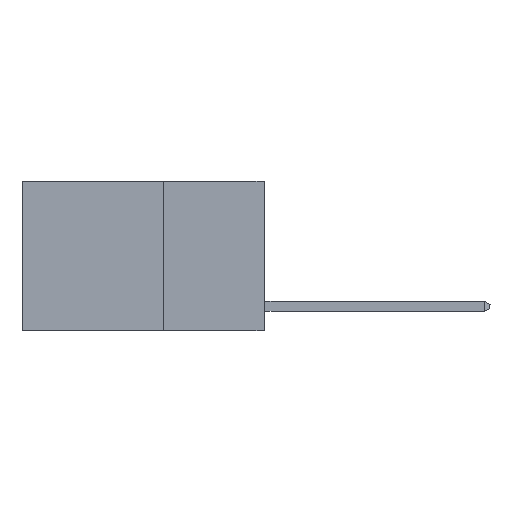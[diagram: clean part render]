
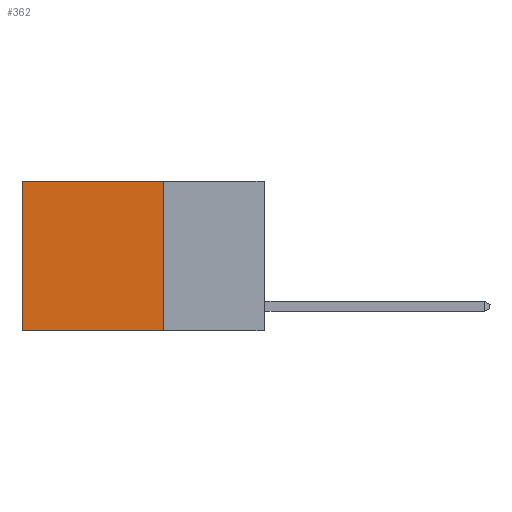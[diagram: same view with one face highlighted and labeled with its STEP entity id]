
A CAD part, left-side view. The second image highlights one B-rep face of the part: STEP entity #362.
In plain terms, the highlighted planar face has unit normal (-1, 0, 0).
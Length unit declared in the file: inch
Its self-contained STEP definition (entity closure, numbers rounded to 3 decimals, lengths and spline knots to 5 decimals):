
#362 = ADVANCED_FACE ( 'NONE', ( #10536 ), #10525, .F. ) ;
#374 = VECTOR ( 'NONE', #8111, 39.37008 ) ;
#999 = VECTOR ( 'NONE', #11682, 39.37008 ) ;
#1847 = ORIENTED_EDGE ( 'NONE', *, *, #6568, .F. ) ;
#2154 = CARTESIAN_POINT ( 'NONE',  ( 0.2625, 0.25, 0. ) ) ;
#2304 = EDGE_CURVE ( 'NONE', #8043, #5341, #3570, .T. ) ;
#2521 = AXIS2_PLACEMENT_3D ( 'NONE', #8917, #4760, #12077 ) ;
#2674 = EDGE_LOOP ( 'NONE', ( #4065, #3410, #1847, #13444 ) ) ;
#3410 = ORIENTED_EDGE ( 'NONE', *, *, #8800, .F. ) ;
#3570 = LINE ( 'NONE', #11479, #9273 ) ;
#4065 = ORIENTED_EDGE ( 'NONE', *, *, #2304, .T. ) ;
#4760 = DIRECTION ( 'NONE',  ( 1., 0., 0. ) ) ;
#5081 = VERTEX_POINT ( 'NONE', #11031 ) ;
#5341 = VERTEX_POINT ( 'NONE', #13574 ) ;
#6568 = EDGE_CURVE ( 'NONE', #11710, #5081, #12863, .T. ) ;
#6842 = CARTESIAN_POINT ( 'NONE',  ( 0.2625, 0.6, 0. ) ) ;
#6962 = CARTESIAN_POINT ( 'NONE',  ( 0.2625, 0.25, 0. ) ) ;
#8043 = VERTEX_POINT ( 'NONE', #6842 ) ;
#8111 = DIRECTION ( 'NONE',  ( 0., 1., 0. ) ) ;
#8800 = EDGE_CURVE ( 'NONE', #5081, #5341, #10043, .T. ) ;
#8917 = CARTESIAN_POINT ( 'NONE',  ( 0.2625, 0.25, 0. ) ) ;
#9273 = VECTOR ( 'NONE', #11380, 39.37008 ) ;
#9442 = LINE ( 'NONE', #6962, #374 ) ;
#10043 = LINE ( 'NONE', #10584, #999 ) ;
#10317 = VECTOR ( 'NONE', #13402, 39.37008 ) ;
#10525 = PLANE ( 'NONE',  #2521 ) ;
#10536 = FACE_OUTER_BOUND ( 'NONE', #2674, .T. ) ;
#10584 = CARTESIAN_POINT ( 'NONE',  ( 0.2625, 0.25, -0.37 ) ) ;
#11031 = CARTESIAN_POINT ( 'NONE',  ( 0.2625, 0.25, -0.37 ) ) ;
#11201 = EDGE_CURVE ( 'NONE', #11710, #8043, #9442, .T. ) ;
#11380 = DIRECTION ( 'NONE',  ( 0., 0., -1. ) ) ;
#11479 = CARTESIAN_POINT ( 'NONE',  ( 0.2625, 0.6, 0. ) ) ;
#11682 = DIRECTION ( 'NONE',  ( 0., 1., 0. ) ) ;
#11710 = VERTEX_POINT ( 'NONE', #2154 ) ;
#12077 = DIRECTION ( 'NONE',  ( 0., 0., -1. ) ) ;
#12367 = CARTESIAN_POINT ( 'NONE',  ( 0.2625, 0.25, 0. ) ) ;
#12863 = LINE ( 'NONE', #12367, #10317 ) ;
#13402 = DIRECTION ( 'NONE',  ( 0., 0., -1. ) ) ;
#13444 = ORIENTED_EDGE ( 'NONE', *, *, #11201, .T. ) ;
#13574 = CARTESIAN_POINT ( 'NONE',  ( 0.2625, 0.6, -0.37 ) ) ;
